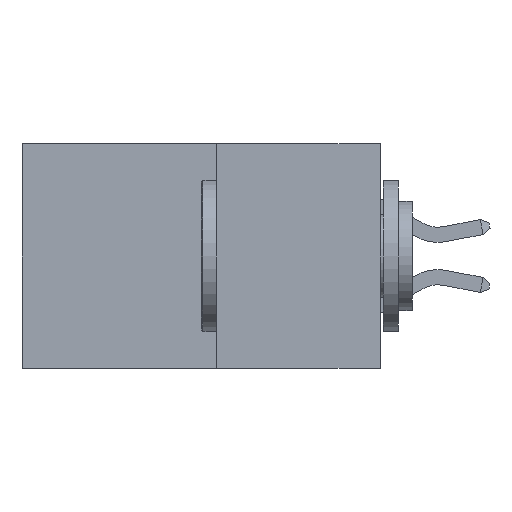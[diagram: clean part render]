
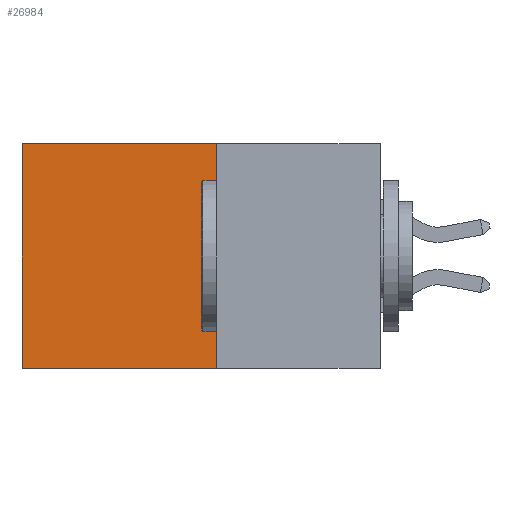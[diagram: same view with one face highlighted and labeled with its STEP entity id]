
A CAD part, left-side view. The second image highlights one B-rep face of the part: STEP entity #26984.
In plain terms, the highlighted planar face has unit normal (-1, 0, 0).
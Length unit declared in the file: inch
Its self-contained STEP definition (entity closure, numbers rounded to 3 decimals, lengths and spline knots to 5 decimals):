
#676 = VERTEX_POINT ( 'NONE', #12952 ) ;
#2494 = DIRECTION ( 'NONE',  ( 0., 0., -1. ) ) ;
#2532 = DIRECTION ( 'NONE',  ( 0., 1., 0. ) ) ;
#3706 = CARTESIAN_POINT ( 'NONE',  ( 0.277, 0.27, 0. ) ) ;
#4372 = LINE ( 'NONE', #3706, #5222 ) ;
#4881 = FACE_OUTER_BOUND ( 'NONE', #10026, .T. ) ;
#4977 = LINE ( 'NONE', #15996, #11305 ) ;
#5222 = VECTOR ( 'NONE', #30175, 39.37008 ) ;
#9942 = LINE ( 'NONE', #33772, #10797 ) ;
#10026 = EDGE_LOOP ( 'NONE', ( #13361, #30929, #33706, #26258 ) ) ;
#10797 = VECTOR ( 'NONE', #28469, 39.37008 ) ;
#11022 = AXIS2_PLACEMENT_3D ( 'NONE', #34327, #18645, #2494 ) ;
#11305 = VECTOR ( 'NONE', #2532, 39.37008 ) ;
#12952 = CARTESIAN_POINT ( 'NONE',  ( 0.277, 0.27, 0. ) ) ;
#13361 = ORIENTED_EDGE ( 'NONE', *, *, #24978, .T. ) ;
#15996 = CARTESIAN_POINT ( 'NONE',  ( 0.277, 0.27, -0.37 ) ) ;
#16979 = EDGE_CURVE ( 'NONE', #25609, #28033, #4977, .T. ) ;
#18258 = CARTESIAN_POINT ( 'NONE',  ( 0.277, 0.27, -0.37 ) ) ;
#18402 = DIRECTION ( 'NONE',  ( 0., 0., -1. ) ) ;
#18645 = DIRECTION ( 'NONE',  ( 1., 0., 0. ) ) ;
#23639 = CARTESIAN_POINT ( 'NONE',  ( 0.277, 0.59, -0.37 ) ) ;
#24803 = VECTOR ( 'NONE', #18402, 39.37008 ) ;
#24978 = EDGE_CURVE ( 'NONE', #26140, #28033, #28320, .T. ) ;
#25609 = VERTEX_POINT ( 'NONE', #18258 ) ;
#26140 = VERTEX_POINT ( 'NONE', #28261 ) ;
#26258 = ORIENTED_EDGE ( 'NONE', *, *, #28095, .T. ) ;
#26379 = PLANE ( 'NONE',  #11022 ) ;
#26806 = EDGE_CURVE ( 'NONE', #676, #25609, #9942, .T. ) ;
#26984 = ADVANCED_FACE ( 'NONE', ( #4881 ), #26379, .F. ) ;
#28033 = VERTEX_POINT ( 'NONE', #32618 ) ;
#28095 = EDGE_CURVE ( 'NONE', #676, #26140, #4372, .T. ) ;
#28261 = CARTESIAN_POINT ( 'NONE',  ( 0.277, 0.59, 0. ) ) ;
#28320 = LINE ( 'NONE', #23639, #24803 ) ;
#28469 = DIRECTION ( 'NONE',  ( 0., 0., -1. ) ) ;
#30175 = DIRECTION ( 'NONE',  ( 0., 1., 0. ) ) ;
#30929 = ORIENTED_EDGE ( 'NONE', *, *, #16979, .F. ) ;
#32618 = CARTESIAN_POINT ( 'NONE',  ( 0.277, 0.59, -0.37 ) ) ;
#33706 = ORIENTED_EDGE ( 'NONE', *, *, #26806, .F. ) ;
#33772 = CARTESIAN_POINT ( 'NONE',  ( 0.277, 0.27, -0.37 ) ) ;
#34327 = CARTESIAN_POINT ( 'NONE',  ( 0.277, 0.27, -0.37 ) ) ;
